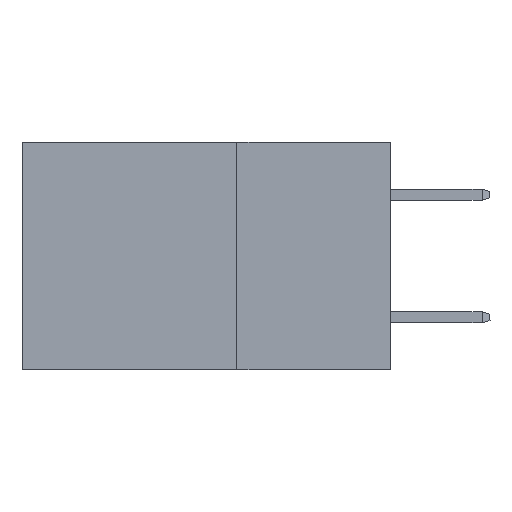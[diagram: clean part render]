
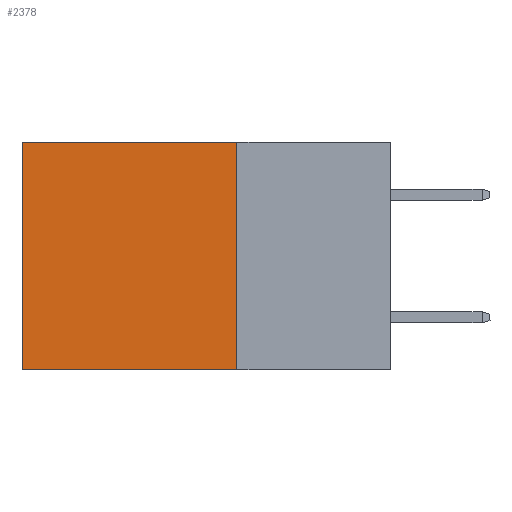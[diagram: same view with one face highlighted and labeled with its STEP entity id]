
A CAD part, left-side view. The second image highlights one B-rep face of the part: STEP entity #2378.
In plain terms, the highlighted planar face has unit normal (-1, 0, 0).
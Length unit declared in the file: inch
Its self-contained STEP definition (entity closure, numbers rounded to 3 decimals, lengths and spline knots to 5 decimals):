
#422 = CARTESIAN_POINT ( 'NONE',  ( 0.2875, 0.25, 0. ) ) ;
#454 = PLANE ( 'NONE',  #10055 ) ;
#614 = CARTESIAN_POINT ( 'NONE',  ( 0.2875, 0.25, 0. ) ) ;
#1683 = VERTEX_POINT ( 'NONE', #8794 ) ;
#2044 = DIRECTION ( 'NONE',  ( 0., 1., 0. ) ) ;
#2255 = CARTESIAN_POINT ( 'NONE',  ( 0.2875, 0.6, -0.37 ) ) ;
#2378 = ADVANCED_FACE ( 'NONE', ( #7271 ), #454, .F. ) ;
#2969 = VECTOR ( 'NONE', #6472, 39.37008 ) ;
#3176 = CARTESIAN_POINT ( 'NONE',  ( 0.2875, 0.6, 0. ) ) ;
#3558 = LINE ( 'NONE', #614, #4736 ) ;
#3729 = DIRECTION ( 'NONE',  ( 0., 0., -1. ) ) ;
#3767 = DIRECTION ( 'NONE',  ( 1., 0., 0. ) ) ;
#3913 = DIRECTION ( 'NONE',  ( 0., 0., -1. ) ) ;
#4000 = VERTEX_POINT ( 'NONE', #5719 ) ;
#4038 = VECTOR ( 'NONE', #8551, 39.37008 ) ;
#4484 = LINE ( 'NONE', #4542, #8403 ) ;
#4542 = CARTESIAN_POINT ( 'NONE',  ( 0.2875, 0.25, -0.37 ) ) ;
#4736 = VECTOR ( 'NONE', #3913, 39.37008 ) ;
#5005 = EDGE_CURVE ( 'NONE', #4000, #9581, #4484, .T. ) ;
#5338 = EDGE_CURVE ( 'NONE', #1683, #9869, #8635, .T. ) ;
#5493 = EDGE_CURVE ( 'NONE', #9869, #9581, #5849, .T. ) ;
#5719 = CARTESIAN_POINT ( 'NONE',  ( 0.2875, 0.25, -0.37 ) ) ;
#5849 = LINE ( 'NONE', #3176, #2969 ) ;
#5974 = CARTESIAN_POINT ( 'NONE',  ( 0.2875, 0.6, 0. ) ) ;
#6472 = DIRECTION ( 'NONE',  ( 0., 0., -1. ) ) ;
#7271 = FACE_OUTER_BOUND ( 'NONE', #8514, .T. ) ;
#7535 = ORIENTED_EDGE ( 'NONE', *, *, #5338, .T. ) ;
#7645 = ORIENTED_EDGE ( 'NONE', *, *, #5493, .T. ) ;
#8403 = VECTOR ( 'NONE', #2044, 39.37008 ) ;
#8514 = EDGE_LOOP ( 'NONE', ( #7645, #10291, #8602, #7535 ) ) ;
#8551 = DIRECTION ( 'NONE',  ( 0., 1., 0. ) ) ;
#8602 = ORIENTED_EDGE ( 'NONE', *, *, #9678, .F. ) ;
#8635 = LINE ( 'NONE', #9372, #4038 ) ;
#8794 = CARTESIAN_POINT ( 'NONE',  ( 0.2875, 0.25, 0. ) ) ;
#9372 = CARTESIAN_POINT ( 'NONE',  ( 0.2875, 0.25, 0. ) ) ;
#9581 = VERTEX_POINT ( 'NONE', #2255 ) ;
#9678 = EDGE_CURVE ( 'NONE', #1683, #4000, #3558, .T. ) ;
#9869 = VERTEX_POINT ( 'NONE', #5974 ) ;
#10055 = AXIS2_PLACEMENT_3D ( 'NONE', #422, #3767, #3729 ) ;
#10291 = ORIENTED_EDGE ( 'NONE', *, *, #5005, .F. ) ;
